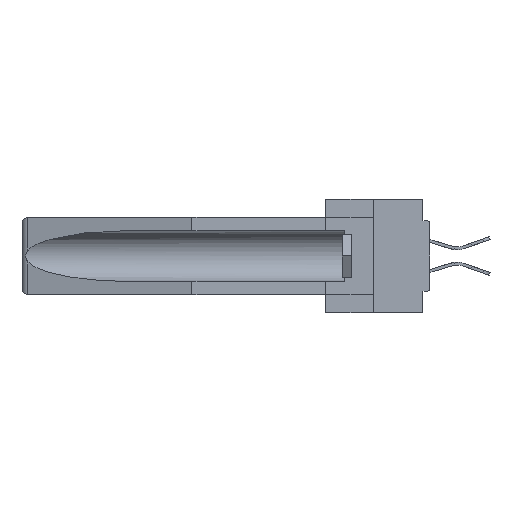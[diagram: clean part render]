
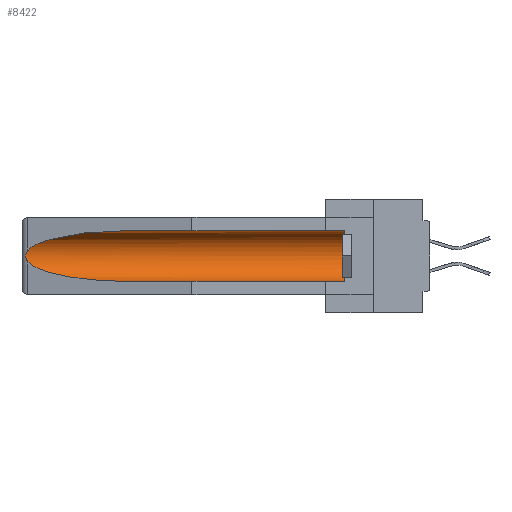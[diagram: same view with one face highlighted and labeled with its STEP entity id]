
A CAD part, left-side view. The second image highlights one B-rep face of the part: STEP entity #8422.
In plain terms, the highlighted cylindrical face has radius 2.857 mm (diameter 5.715 mm), a partial arc.
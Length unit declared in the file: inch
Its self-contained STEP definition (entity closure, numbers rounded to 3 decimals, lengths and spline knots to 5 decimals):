
#553 = CARTESIAN_POINT ( 'NONE',  ( 0.26597, 1.5296, -0.19026 ) ) ;
#728 = CARTESIAN_POINT ( 'NONE',  ( 0.155, -0.30754, -0.059 ) ) ;
#3827 = CARTESIAN_POINT ( 'NONE',  ( 0.155, 1.07973, -0.059 ) ) ;
#4197 = CARTESIAN_POINT ( 'NONE',  ( 0.26654, 1.53092, -0.15636 ) ) ;
#5671 = DIRECTION ( 'NONE',  ( 0., 1., 0. ) ) ;
#5695 = B_SPLINE_CURVE_WITH_KNOTS ( 'NONE', 3,
 ( #37174, #25841, #4197, #33071, #15459, #33404, #44473, #11518, #553, #15614 ),
 .UNSPECIFIED., .F., .F.,
 ( 4, 2, 2, 2, 4 ),
 ( 0., 0.00029, 0.00058, 0.00087, 0.00117 ),
 .UNSPECIFIED. ) ;
#6063 = EDGE_CURVE ( 'NONE', #42744, #32540, #32159, .T. ) ;
#6173 = ORIENTED_EDGE ( 'NONE', *, *, #26454, .F. ) ;
#6979 = CARTESIAN_POINT ( 'NONE',  ( 0.26537, 1.52718, -0.14972 ) ) ;
#8422 = ADVANCED_FACE ( 'NONE', ( #22015 ), #10207, .F. ) ;
#9263 = LINE ( 'NONE', #728, #40198 ) ;
#9653 = VERTEX_POINT ( 'NONE', #14237 ) ;
#9778 = EDGE_CURVE ( 'NONE', #9653, #40541, #9263, .T. ) ;
#10207 = CYLINDRICAL_SURFACE ( 'NONE', #40877, 0.1125 ) ;
#10234 = CARTESIAN_POINT ( 'NONE',  ( 0.21114, 1.30732, -0.059 ) ) ;
#11387 = DIRECTION ( 'NONE',  ( 0., 1., 0. ) ) ;
#11518 = CARTESIAN_POINT ( 'NONE',  ( 0.26655, 1.53094, -0.18657 ) ) ;
#14237 = CARTESIAN_POINT ( 'NONE',  ( 0.155, 0.126, -0.059 ) ) ;
#14430 = DIRECTION ( 'NONE',  ( 0., 0., 1. ) ) ;
#15212 = ORIENTED_EDGE ( 'NONE', *, *, #28481, .T. ) ;
#15459 = CARTESIAN_POINT ( 'NONE',  ( 0.2675, 1.53308, -0.16763 ) ) ;
#15614 = CARTESIAN_POINT ( 'NONE',  ( 0.26537, 1.52718, -0.19328 ) ) ;
#16968 = DIRECTION ( 'NONE',  ( 0., -1., 0. ) ) ;
#17185 = ORIENTED_EDGE ( 'NONE', *, *, #27661, .T. ) ;
#18978 = LINE ( 'NONE', #30630, #28578 ) ;
#19315 = CARTESIAN_POINT ( 'NONE',  ( 0.155, 1.07973, -0.284 ) ) ;
#20700 = DIRECTION ( 'NONE',  ( 0., 1., 0. ) ) ;
#21787 = CARTESIAN_POINT ( 'NONE',  ( 0.155, 1.07973, -0.059 ) ) ;
#22015 = FACE_OUTER_BOUND ( 'NONE', #41375, .T. ) ;
#24195 = CARTESIAN_POINT ( 'NONE',  ( 0.25451, 1.48313, -0.24835 ) ) ;
#24323 = EDGE_CURVE ( 'NONE', #24870, #9653, #26584, .T. ) ;
#24357 = CARTESIAN_POINT ( 'NONE',  ( 0.26537, 1.52718, -0.19328 ) ) ;
#24870 = VERTEX_POINT ( 'NONE', #28834 ) ;
#25815 = ORIENTED_EDGE ( 'NONE', *, *, #24323, .T. ) ;
#25841 = CARTESIAN_POINT ( 'NONE',  ( 0.26597, 1.52961, -0.15275 ) ) ;
#26454 = EDGE_CURVE ( 'NONE', #24870, #32540, #18978, .T. ) ;
#26584 = CIRCLE ( 'NONE', #38438, 0.1125 ) ;
#27661 = EDGE_CURVE ( 'NONE', #40541, #31635, #40540, .T. ) ;
#28339 = CARTESIAN_POINT ( 'NONE',  ( 0.25451, 1.48313, -0.09465 ) ) ;
#28481 = EDGE_CURVE ( 'NONE', #31635, #42744, #5695, .T. ) ;
#28578 = VECTOR ( 'NONE', #5671, 39.37008 ) ;
#28834 = CARTESIAN_POINT ( 'NONE',  ( 0.155, 0.126, -0.284 ) ) ;
#30193 = CARTESIAN_POINT ( 'NONE',  ( 0.26537, 1.52718, -0.19328 ) ) ;
#30630 = CARTESIAN_POINT ( 'NONE',  ( 0.155, -0.30754, -0.284 ) ) ;
#31635 = VERTEX_POINT ( 'NONE', #45892 ) ;
#32159 =( BOUNDED_CURVE ( )  B_SPLINE_CURVE ( 3, ( #24357, #24195, #35041, #34731 ),
 .UNSPECIFIED., .F., .F. ) 
 B_SPLINE_CURVE_WITH_KNOTS ( ( 4, 4 ),
 ( 0.1948, 1.5708 ),
 .UNSPECIFIED. ) 
 CURVE ( )  GEOMETRIC_REPRESENTATION_ITEM ( )  RATIONAL_B_SPLINE_CURVE ( ( 1., 0.848, 0.848, 1. ) ) 
 REPRESENTATION_ITEM ( '' )  );
#32540 = VERTEX_POINT ( 'NONE', #19315 ) ;
#33071 = CARTESIAN_POINT ( 'NONE',  ( 0.2673, 1.5327, -0.16383 ) ) ;
#33257 = CARTESIAN_POINT ( 'NONE',  ( 0.155, 0.126, -0.1715 ) ) ;
#33404 = CARTESIAN_POINT ( 'NONE',  ( 0.2675, 1.53308, -0.17534 ) ) ;
#34731 = CARTESIAN_POINT ( 'NONE',  ( 0.155, 1.07973, -0.284 ) ) ;
#35041 = CARTESIAN_POINT ( 'NONE',  ( 0.21114, 1.30732, -0.284 ) ) ;
#37174 = CARTESIAN_POINT ( 'NONE',  ( 0.26537, 1.52718, -0.14972 ) ) ;
#38438 = AXIS2_PLACEMENT_3D ( 'NONE', #33257, #16968, #14430 ) ;
#38937 = CARTESIAN_POINT ( 'NONE',  ( 0.155, -0.30754, -0.1715 ) ) ;
#40198 = VECTOR ( 'NONE', #11387, 39.37008 ) ;
#40540 =( BOUNDED_CURVE ( )  B_SPLINE_CURVE ( 3, ( #3827, #10234, #28339, #6979 ),
 .UNSPECIFIED., .F., .F. ) 
 B_SPLINE_CURVE_WITH_KNOTS ( ( 4, 4 ),
 ( 4.71239, 6.08839 ),
 .UNSPECIFIED. ) 
 CURVE ( )  GEOMETRIC_REPRESENTATION_ITEM ( )  RATIONAL_B_SPLINE_CURVE ( ( 1., 0.848, 0.848, 1. ) ) 
 REPRESENTATION_ITEM ( '' )  );
#40541 = VERTEX_POINT ( 'NONE', #21787 ) ;
#40877 = AXIS2_PLACEMENT_3D ( 'NONE', #38937, #20700, #46386 ) ;
#41375 = EDGE_LOOP ( 'NONE', ( #17185, #15212, #43177, #6173, #25815, #46189 ) ) ;
#42744 = VERTEX_POINT ( 'NONE', #30193 ) ;
#43177 = ORIENTED_EDGE ( 'NONE', *, *, #6063, .T. ) ;
#44473 = CARTESIAN_POINT ( 'NONE',  ( 0.2673, 1.53269, -0.17917 ) ) ;
#45892 = CARTESIAN_POINT ( 'NONE',  ( 0.26537, 1.52718, -0.14972 ) ) ;
#46189 = ORIENTED_EDGE ( 'NONE', *, *, #9778, .T. ) ;
#46386 = DIRECTION ( 'NONE',  ( 0., 0., 1. ) ) ;
